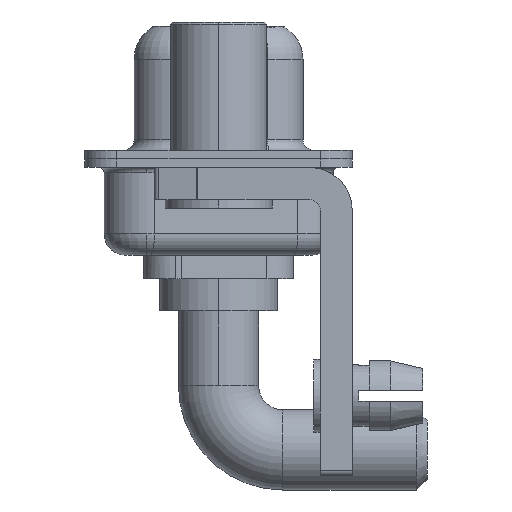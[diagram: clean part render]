
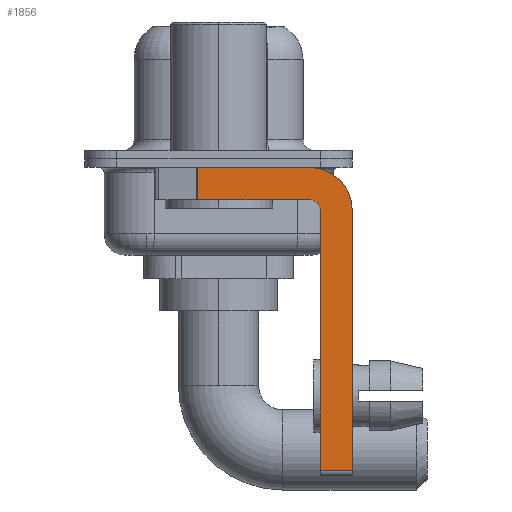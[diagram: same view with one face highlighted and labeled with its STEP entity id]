
A CAD part, left-side view. The second image highlights one B-rep face of the part: STEP entity #1856.
In plain terms, the highlighted planar face has unit normal (-1, 0, 0).
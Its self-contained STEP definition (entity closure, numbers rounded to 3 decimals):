
#55 = LINE ( 'NONE', #6307, #1918 ) ;
#99 = ORIENTED_EDGE ( 'NONE', *, *, #8735, .F. ) ;
#134 = DIRECTION ( 'NONE',  ( 0., -1., 0. ) ) ;
#454 = CIRCLE ( 'NONE', #14397, 0.5 ) ;
#476 = EDGE_CURVE ( 'NONE', #8257, #9561, #772, .T. ) ;
#730 = VERTEX_POINT ( 'NONE', #15197 ) ;
#772 = LINE ( 'NONE', #9658, #15334 ) ;
#899 = LINE ( 'NONE', #9864, #7922 ) ;
#942 = CARTESIAN_POINT ( 'NONE',  ( -2.9, -4.25, -2.4 ) ) ;
#1366 = AXIS2_PLACEMENT_3D ( 'NONE', #9931, #11252, #6223 ) ;
#1731 = VERTEX_POINT ( 'NONE', #12411 ) ;
#1856 = ADVANCED_FACE ( 'NONE', ( #2433 ), #4910, .F. ) ;
#1918 = VECTOR ( 'NONE', #134, 1000. ) ;
#2091 = DIRECTION ( 'NONE',  ( 0., 0., 1. ) ) ;
#2164 = VECTOR ( 'NONE', #4571, 1000. ) ;
#2235 = CARTESIAN_POINT ( 'NONE',  ( -2.9, -4.25, -1.9 ) ) ;
#2333 = DIRECTION ( 'NONE',  ( -1., 0., 0. ) ) ;
#2433 = FACE_OUTER_BOUND ( 'NONE', #6059, .T. ) ;
#2684 = CARTESIAN_POINT ( 'NONE',  ( -2.9, 0.978, -1.9 ) ) ;
#3306 = ORIENTED_EDGE ( 'NONE', *, *, #12468, .F. ) ;
#3715 = ORIENTED_EDGE ( 'NONE', *, *, #10110, .F. ) ;
#3802 = EDGE_CURVE ( 'NONE', #8257, #6440, #9433, .T. ) ;
#3837 = VECTOR ( 'NONE', #15651, 1000. ) ;
#4235 = CARTESIAN_POINT ( 'NONE',  ( -2.9, -6.25, -14.55 ) ) ;
#4571 = DIRECTION ( 'NONE',  ( 0., -1., 0. ) ) ;
#4624 = AXIS2_PLACEMENT_3D ( 'NONE', #15606, #6792, #13229 ) ;
#4910 = PLANE ( 'NONE',  #1366 ) ;
#5032 = VERTEX_POINT ( 'NONE', #11750 ) ;
#5203 = LINE ( 'NONE', #9235, #13771 ) ;
#5770 = ORIENTED_EDGE ( 'NONE', *, *, #13241, .F. ) ;
#6059 = EDGE_LOOP ( 'NONE', ( #3306, #12724, #10883, #99, #8344, #6422, #5770, #3715 ) ) ;
#6223 = DIRECTION ( 'NONE',  ( 0., 0., -1. ) ) ;
#6307 = CARTESIAN_POINT ( 'NONE',  ( -2.9, 3., -0.4 ) ) ;
#6389 = VERTEX_POINT ( 'NONE', #2684 ) ;
#6422 = ORIENTED_EDGE ( 'NONE', *, *, #3802, .T. ) ;
#6440 = VERTEX_POINT ( 'NONE', #4235 ) ;
#6455 = CIRCLE ( 'NONE', #4624, 2. ) ;
#6761 = CARTESIAN_POINT ( 'NONE',  ( -2.9, -4.25, -1.9 ) ) ;
#6792 = DIRECTION ( 'NONE',  ( 1., 0., 0. ) ) ;
#6931 = LINE ( 'NONE', #6761, #3837 ) ;
#7221 = DIRECTION ( 'NONE',  ( 0., 0., -1. ) ) ;
#7922 = VECTOR ( 'NONE', #7221, 1000. ) ;
#8257 = VERTEX_POINT ( 'NONE', #14316 ) ;
#8344 = ORIENTED_EDGE ( 'NONE', *, *, #476, .F. ) ;
#8366 = CARTESIAN_POINT ( 'NONE',  ( -2.9, -4.25, -14.55 ) ) ;
#8735 = EDGE_CURVE ( 'NONE', #9561, #14744, #454, .T. ) ;
#9235 = CARTESIAN_POINT ( 'NONE',  ( -2.9, 0.978, -1.9 ) ) ;
#9433 = LINE ( 'NONE', #8366, #2164 ) ;
#9561 = VERTEX_POINT ( 'NONE', #10684 ) ;
#9658 = CARTESIAN_POINT ( 'NONE',  ( -2.9, -4.75, -14.8 ) ) ;
#9864 = CARTESIAN_POINT ( 'NONE',  ( -2.9, -6.25, -2.4 ) ) ;
#9931 = CARTESIAN_POINT ( 'NONE',  ( -2.9, -4.25, -2.4 ) ) ;
#10110 = EDGE_CURVE ( 'NONE', #730, #5032, #6455, .T. ) ;
#10471 = DIRECTION ( 'NONE',  ( 0., 0., -1. ) ) ;
#10684 = CARTESIAN_POINT ( 'NONE',  ( -2.9, -4.75, -2.4 ) ) ;
#10801 = EDGE_CURVE ( 'NONE', #14744, #6389, #6931, .T. ) ;
#10883 = ORIENTED_EDGE ( 'NONE', *, *, #10801, .F. ) ;
#10978 = DIRECTION ( 'NONE',  ( 0., 0., 1. ) ) ;
#11252 = DIRECTION ( 'NONE',  ( 1., 0., 0. ) ) ;
#11750 = CARTESIAN_POINT ( 'NONE',  ( -2.9, -6.25, -2.4 ) ) ;
#12411 = CARTESIAN_POINT ( 'NONE',  ( -2.9, 0.978, -0.4 ) ) ;
#12468 = EDGE_CURVE ( 'NONE', #1731, #730, #55, .T. ) ;
#12724 = ORIENTED_EDGE ( 'NONE', *, *, #14449, .T. ) ;
#13229 = DIRECTION ( 'NONE',  ( 0., 0., -1. ) ) ;
#13241 = EDGE_CURVE ( 'NONE', #5032, #6440, #899, .T. ) ;
#13771 = VECTOR ( 'NONE', #10471, 1000. ) ;
#14316 = CARTESIAN_POINT ( 'NONE',  ( -2.9, -4.75, -14.55 ) ) ;
#14397 = AXIS2_PLACEMENT_3D ( 'NONE', #942, #2333, #2091 ) ;
#14449 = EDGE_CURVE ( 'NONE', #1731, #6389, #5203, .T. ) ;
#14744 = VERTEX_POINT ( 'NONE', #2235 ) ;
#15197 = CARTESIAN_POINT ( 'NONE',  ( -2.9, -4.25, -0.4 ) ) ;
#15334 = VECTOR ( 'NONE', #10978, 1000. ) ;
#15606 = CARTESIAN_POINT ( 'NONE',  ( -2.9, -4.25, -2.4 ) ) ;
#15651 = DIRECTION ( 'NONE',  ( 0., 1., 0. ) ) ;
